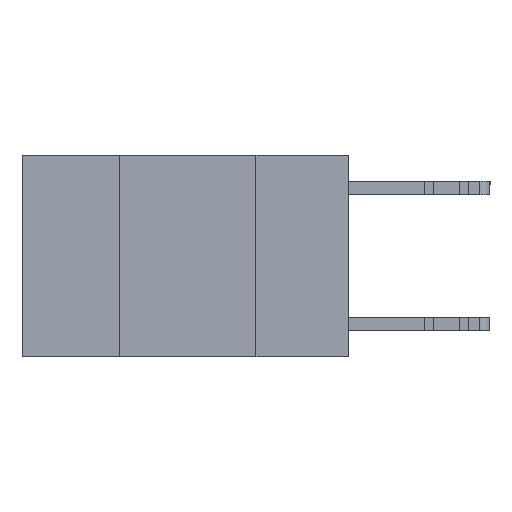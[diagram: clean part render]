
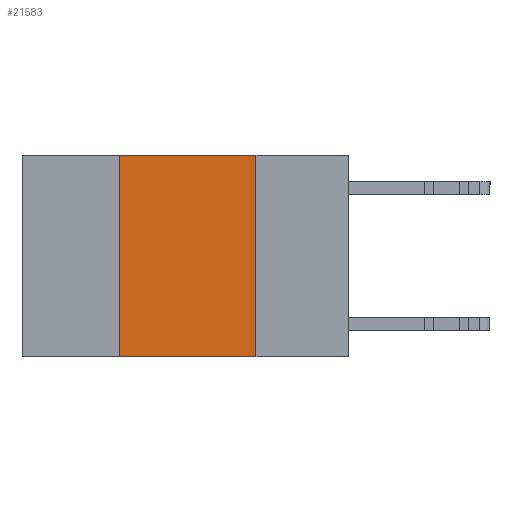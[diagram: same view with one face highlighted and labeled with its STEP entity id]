
A CAD part, left-side view. The second image highlights one B-rep face of the part: STEP entity #21583.
In plain terms, the highlighted planar face has unit normal (-1, 0, 0).
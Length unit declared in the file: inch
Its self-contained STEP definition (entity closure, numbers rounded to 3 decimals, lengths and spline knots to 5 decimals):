
#331 = CARTESIAN_POINT ( 'NONE',  ( 0., 0.6, 0. ) ) ;
#1452 = ORIENTED_EDGE ( 'NONE', *, *, #5553, .F. ) ;
#2656 = AXIS2_PLACEMENT_3D ( 'NONE', #22665, #15453, #18339 ) ;
#2667 = EDGE_LOOP ( 'NONE', ( #27471, #1452, #11431, #14746 ) ) ;
#3561 = VECTOR ( 'NONE', #29200, 39.37008 ) ;
#3767 = PLANE ( 'NONE',  #2656 ) ;
#5553 = EDGE_CURVE ( 'NONE', #19076, #15032, #22916, .T. ) ;
#5989 = CARTESIAN_POINT ( 'NONE',  ( 0., 0.42, 0. ) ) ;
#7263 = LINE ( 'NONE', #29223, #23063 ) ;
#8056 = LINE ( 'NONE', #5989, #19921 ) ;
#8171 = EDGE_CURVE ( 'NONE', #16935, #30164, #19411, .T. ) ;
#9642 = CARTESIAN_POINT ( 'NONE',  ( 0., 0.6, -0.37 ) ) ;
#10126 = EDGE_CURVE ( 'NONE', #16935, #19076, #8056, .T. ) ;
#10651 = FACE_OUTER_BOUND ( 'NONE', #2667, .T. ) ;
#10749 = DIRECTION ( 'NONE',  ( 0., -1., 0. ) ) ;
#11431 = ORIENTED_EDGE ( 'NONE', *, *, #10126, .F. ) ;
#11504 = CARTESIAN_POINT ( 'NONE',  ( 0., 0.42, 0. ) ) ;
#13190 = DIRECTION ( 'NONE',  ( 0., 0., 1. ) ) ;
#13717 = CARTESIAN_POINT ( 'NONE',  ( 0., 0.17, 0. ) ) ;
#14746 = ORIENTED_EDGE ( 'NONE', *, *, #8171, .T. ) ;
#15032 = VERTEX_POINT ( 'NONE', #13717 ) ;
#15453 = DIRECTION ( 'NONE',  ( 1., 0., 0. ) ) ;
#16935 = VERTEX_POINT ( 'NONE', #23638 ) ;
#18339 = DIRECTION ( 'NONE',  ( 0., 0., -1. ) ) ;
#19076 = VERTEX_POINT ( 'NONE', #11504 ) ;
#19411 = LINE ( 'NONE', #9642, #3561 ) ;
#19739 = EDGE_CURVE ( 'NONE', #15032, #30164, #7263, .T. ) ;
#19921 = VECTOR ( 'NONE', #13190, 39.37008 ) ;
#20893 = VECTOR ( 'NONE', #10749, 39.37008 ) ;
#21583 = ADVANCED_FACE ( 'NONE', ( #10651 ), #3767, .F. ) ;
#22665 = CARTESIAN_POINT ( 'NONE',  ( 0., 0.6, 0. ) ) ;
#22916 = LINE ( 'NONE', #331, #20893 ) ;
#23063 = VECTOR ( 'NONE', #24391, 39.37008 ) ;
#23638 = CARTESIAN_POINT ( 'NONE',  ( 0., 0.42, -0.37 ) ) ;
#24034 = CARTESIAN_POINT ( 'NONE',  ( 0., 0.17, -0.37 ) ) ;
#24391 = DIRECTION ( 'NONE',  ( 0., 0., -1. ) ) ;
#27471 = ORIENTED_EDGE ( 'NONE', *, *, #19739, .F. ) ;
#29200 = DIRECTION ( 'NONE',  ( 0., -1., 0. ) ) ;
#29223 = CARTESIAN_POINT ( 'NONE',  ( 0., 0.17, 0. ) ) ;
#30164 = VERTEX_POINT ( 'NONE', #24034 ) ;
